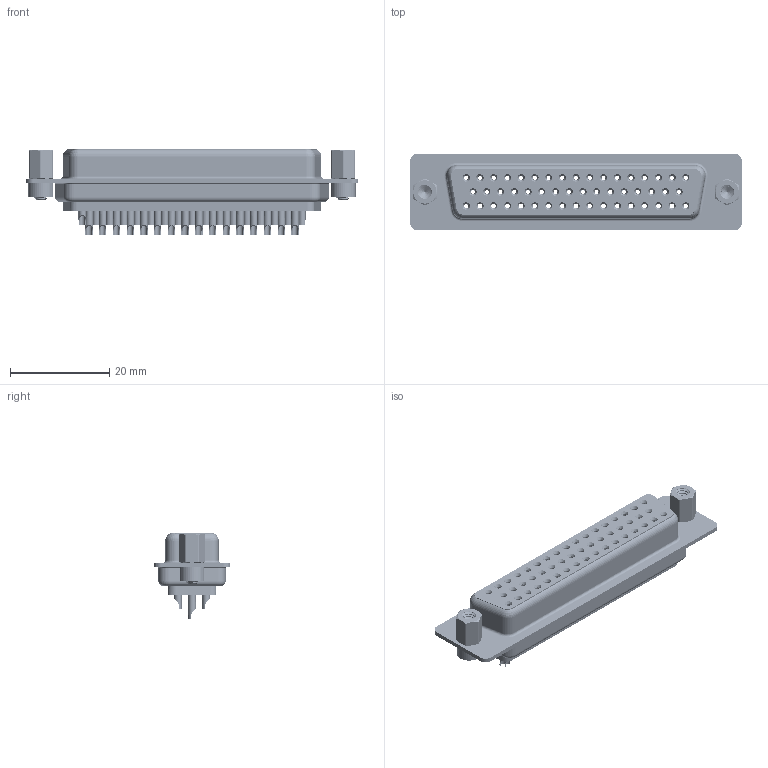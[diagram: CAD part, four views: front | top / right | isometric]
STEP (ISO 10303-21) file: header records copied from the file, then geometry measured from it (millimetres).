
FILE_DESCRIPTION (( 'STEP AP203' ), '1' );
FILE_NAME ('628-050-222-543.STEP', '2018-10-20T07:46:41', ( '' ), ( '' ), 'SwSTEP 2.0', 'SolidWorks 2016', '' );
FILE_SCHEMA (( 'CONFIG_CONTROL_DESIGN' ));
Length unit declared in the file: millimetre
Products named in the file (9): 628 4-40 Hex Standoff; 628-050-222-543; 628 Housing_50 LP; 628 Shell Front_50 Contacts; 628 Shell Rear_50 Contacts; 628 Contact Row 1_22L; 628 Contact Row 2_22M; 628 Contact Row 3_22L; 628 4-40 Threaded Rivet
Assembly tree (41 placements, depth 2):
  628-050-222-543
    628 Housing_50 LP
    628 Shell Front_50 Contacts
    628 Shell Rear_50 Contacts
    628 Contact Row 1_22L  x17
    628 Contact Row 2_22M  x16
    628 Contact Row 3_22L
    628 4-40 Threaded Rivet  x2
    628 4-40 Hex Standoff  x2
Bounding box: 67 x 15.4 x 17.35 mm (x, y, z)
Volume: 6848.4 mm3; surface area: 14614.6 mm2
Topology: 41 solids, 41 shells, 3639 faces, 9167 edges, 5771 vertices
Faces by surface type: cylinder 1187, plane 851, bspline 698, torus 675, cone 228
Entity records: 42711 total; most frequent: CARTESIAN_POINT 13212, DIRECTION 6103, ORIENTED_EDGE 5542, EDGE_CURVE 2771, AXIS2_PLACEMENT_3D 2571, VERTEX_POINT 1761, EDGE_LOOP 1462, CIRCLE 1409
